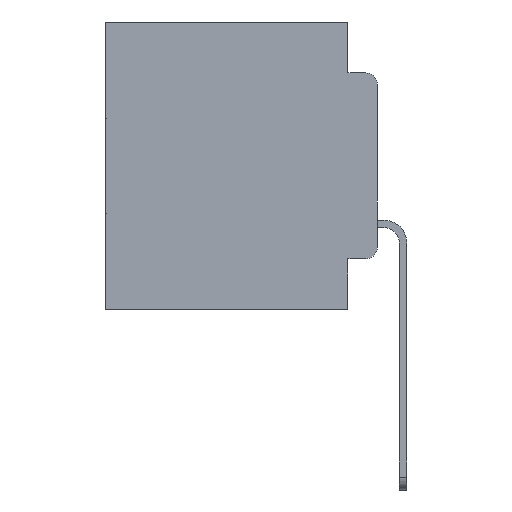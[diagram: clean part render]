
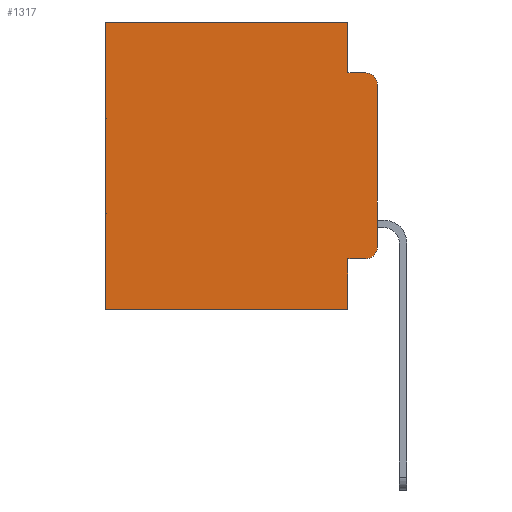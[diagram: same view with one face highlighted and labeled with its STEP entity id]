
A CAD part, left-side view. The second image highlights one B-rep face of the part: STEP entity #1317.
In plain terms, the highlighted planar face has unit normal (-1, 0, 0).
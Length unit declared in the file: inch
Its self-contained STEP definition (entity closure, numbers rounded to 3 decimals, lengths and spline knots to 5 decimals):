
#27 = ORIENTED_EDGE ( 'NONE', *, *, #9074, .F. ) ;
#523 = ORIENTED_EDGE ( 'NONE', *, *, #23071, .T. ) ;
#533 = LINE ( 'NONE', #13214, #12300 ) ;
#595 = PLANE ( 'NONE',  #1234 ) ;
#698 = LINE ( 'NONE', #5571, #6999 ) ;
#915 = VERTEX_POINT ( 'NONE', #11522 ) ;
#976 = CARTESIAN_POINT ( 'NONE',  ( 0.298, 0., 0. ) ) ;
#1234 = AXIS2_PLACEMENT_3D ( 'NONE', #12763, #13470, #25174 ) ;
#1317 = ADVANCED_FACE ( 'NONE', ( #22589 ), #595, .F. ) ;
#2209 = AXIS2_PLACEMENT_3D ( 'NONE', #27440, #13765, #29554 ) ;
#2305 = AXIS2_PLACEMENT_3D ( 'NONE', #3712, #19907, #6027 ) ;
#2833 = DIRECTION ( 'NONE',  ( 0., 0., -1. ) ) ;
#2961 = VERTEX_POINT ( 'NONE', #17094 ) ;
#3063 = VECTOR ( 'NONE', #24568, 39.37008 ) ;
#3192 = ORIENTED_EDGE ( 'NONE', *, *, #5990, .T. ) ;
#3416 = DIRECTION ( 'NONE',  ( 0., 1., 0. ) ) ;
#3712 = CARTESIAN_POINT ( 'NONE',  ( 0.298, 0.02, -0.3915 ) ) ;
#3918 = DIRECTION ( 'NONE',  ( 0., 0., -1. ) ) ;
#4257 = ORIENTED_EDGE ( 'NONE', *, *, #10603, .T. ) ;
#4367 = CIRCLE ( 'NONE', #2209, 0.02 ) ;
#5413 = ORIENTED_EDGE ( 'NONE', *, *, #21519, .F. ) ;
#5511 = LINE ( 'NONE', #22450, #23237 ) ;
#5571 = CARTESIAN_POINT ( 'NONE',  ( 0.298, 0.051, -0.0885 ) ) ;
#5875 = CARTESIAN_POINT ( 'NONE',  ( 0.298, 0., -0.3915 ) ) ;
#5990 = EDGE_CURVE ( 'NONE', #8309, #24152, #10368, .T. ) ;
#6022 = VERTEX_POINT ( 'NONE', #15402 ) ;
#6027 = DIRECTION ( 'NONE',  ( 0., 0., -1. ) ) ;
#6032 = LINE ( 'NONE', #976, #11460 ) ;
#6454 = LINE ( 'NONE', #19912, #23461 ) ;
#6607 = VERTEX_POINT ( 'NONE', #12847 ) ;
#6999 = VECTOR ( 'NONE', #7868, 39.37008 ) ;
#7513 = CARTESIAN_POINT ( 'NONE',  ( 0.298, 0., 0. ) ) ;
#7547 = EDGE_CURVE ( 'NONE', #13119, #8309, #14750, .T. ) ;
#7868 = DIRECTION ( 'NONE',  ( 0., -1., 0. ) ) ;
#8309 = VERTEX_POINT ( 'NONE', #17470 ) ;
#8502 = DIRECTION ( 'NONE',  ( 0., 0., -1. ) ) ;
#9074 = EDGE_CURVE ( 'NONE', #13119, #6022, #5511, .T. ) ;
#10368 = CIRCLE ( 'NONE', #2305, 0.02 ) ;
#10572 = CARTESIAN_POINT ( 'NONE',  ( 0.298, 0.051, -0.4115 ) ) ;
#10603 = EDGE_CURVE ( 'NONE', #22594, #6607, #533, .T. ) ;
#11460 = VECTOR ( 'NONE', #3416, 39.37008 ) ;
#11522 = CARTESIAN_POINT ( 'NONE',  ( 0.298, 0., -0.1085 ) ) ;
#11722 = ORIENTED_EDGE ( 'NONE', *, *, #25920, .F. ) ;
#12300 = VECTOR ( 'NONE', #8502, 39.37008 ) ;
#12763 = CARTESIAN_POINT ( 'NONE',  ( 0.298, 0., 0. ) ) ;
#12847 = CARTESIAN_POINT ( 'NONE',  ( 0.298, 0.473, -0.5 ) ) ;
#13115 = DIRECTION ( 'NONE',  ( 0., -1., 0. ) ) ;
#13119 = VERTEX_POINT ( 'NONE', #10572 ) ;
#13214 = CARTESIAN_POINT ( 'NONE',  ( 0.298, 0.473, 0. ) ) ;
#13470 = DIRECTION ( 'NONE',  ( 1., 0., 0. ) ) ;
#13765 = DIRECTION ( 'NONE',  ( -1., 0., 0. ) ) ;
#14750 = LINE ( 'NONE', #17754, #20122 ) ;
#15364 = EDGE_CURVE ( 'NONE', #2961, #20372, #6454, .T. ) ;
#15402 = CARTESIAN_POINT ( 'NONE',  ( 0.298, 0.051, -0.5 ) ) ;
#15409 = DIRECTION ( 'NONE',  ( 0., 0., -1. ) ) ;
#16912 = VECTOR ( 'NONE', #2833, 39.37008 ) ;
#17030 = ORIENTED_EDGE ( 'NONE', *, *, #19452, .T. ) ;
#17094 = CARTESIAN_POINT ( 'NONE',  ( 0.298, 0.051, 0. ) ) ;
#17280 = VERTEX_POINT ( 'NONE', #26790 ) ;
#17470 = CARTESIAN_POINT ( 'NONE',  ( 0.298, 0.02, -0.4115 ) ) ;
#17702 = CARTESIAN_POINT ( 'NONE',  ( 0.298, 0., -0.5 ) ) ;
#17754 = CARTESIAN_POINT ( 'NONE',  ( 0.298, 0.051, -0.4115 ) ) ;
#19452 = EDGE_CURVE ( 'NONE', #2961, #22594, #6032, .T. ) ;
#19907 = DIRECTION ( 'NONE',  ( -1., 0., 0. ) ) ;
#19912 = CARTESIAN_POINT ( 'NONE',  ( 0.298, 0.051, 0. ) ) ;
#20122 = VECTOR ( 'NONE', #13115, 39.37008 ) ;
#20372 = VERTEX_POINT ( 'NONE', #28651 ) ;
#20933 = ORIENTED_EDGE ( 'NONE', *, *, #7547, .T. ) ;
#21519 = EDGE_CURVE ( 'NONE', #20372, #17280, #698, .T. ) ;
#21560 = LINE ( 'NONE', #17702, #3063 ) ;
#22450 = CARTESIAN_POINT ( 'NONE',  ( 0.298, 0.051, 0. ) ) ;
#22589 = FACE_OUTER_BOUND ( 'NONE', #29376, .T. ) ;
#22594 = VERTEX_POINT ( 'NONE', #25614 ) ;
#22999 = LINE ( 'NONE', #7513, #16912 ) ;
#23071 = EDGE_CURVE ( 'NONE', #915, #17280, #4367, .T. ) ;
#23143 = ORIENTED_EDGE ( 'NONE', *, *, #28981, .F. ) ;
#23237 = VECTOR ( 'NONE', #3918, 39.37008 ) ;
#23461 = VECTOR ( 'NONE', #15409, 39.37008 ) ;
#24152 = VERTEX_POINT ( 'NONE', #5875 ) ;
#24568 = DIRECTION ( 'NONE',  ( 0., 1., 0. ) ) ;
#25174 = DIRECTION ( 'NONE',  ( 0., 0., -1. ) ) ;
#25614 = CARTESIAN_POINT ( 'NONE',  ( 0.298, 0.473, 0. ) ) ;
#25920 = EDGE_CURVE ( 'NONE', #6022, #6607, #21560, .T. ) ;
#26667 = ORIENTED_EDGE ( 'NONE', *, *, #15364, .F. ) ;
#26790 = CARTESIAN_POINT ( 'NONE',  ( 0.298, 0.02, -0.0885 ) ) ;
#27440 = CARTESIAN_POINT ( 'NONE',  ( 0.298, 0.02, -0.1085 ) ) ;
#28651 = CARTESIAN_POINT ( 'NONE',  ( 0.298, 0.051, -0.0885 ) ) ;
#28981 = EDGE_CURVE ( 'NONE', #915, #24152, #22999, .T. ) ;
#29376 = EDGE_LOOP ( 'NONE', ( #23143, #523, #5413, #26667, #17030, #4257, #11722, #27, #20933, #3192 ) ) ;
#29554 = DIRECTION ( 'NONE',  ( 0., 0., -1. ) ) ;
